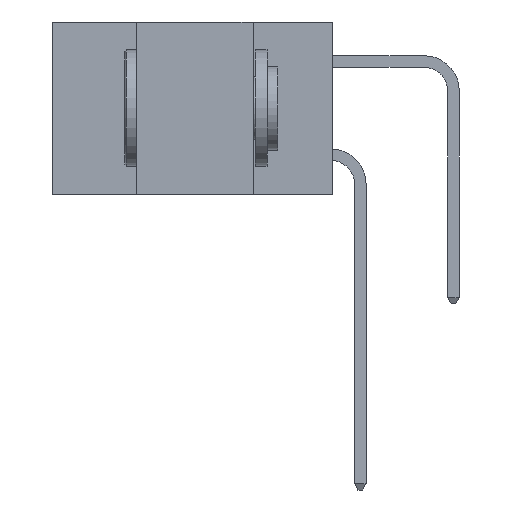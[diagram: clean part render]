
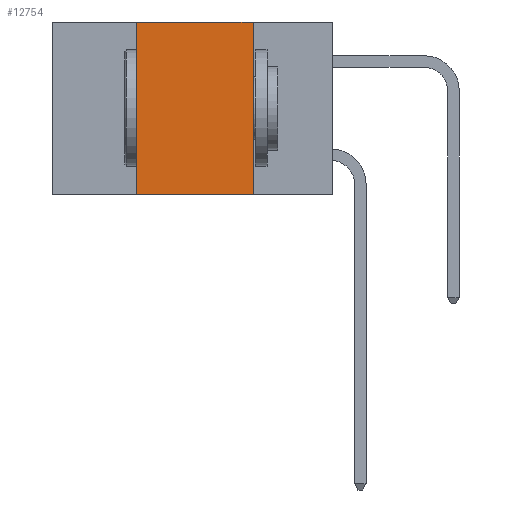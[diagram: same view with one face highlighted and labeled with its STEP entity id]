
A CAD part, left-side view. The second image highlights one B-rep face of the part: STEP entity #12754.
In plain terms, the highlighted planar face has unit normal (-1, 0, 0).
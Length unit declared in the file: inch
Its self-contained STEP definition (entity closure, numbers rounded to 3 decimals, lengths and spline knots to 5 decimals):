
#798 = EDGE_CURVE ( 'NONE', #11779, #3579, #15846, .T. ) ;
#1297 = CARTESIAN_POINT ( 'NONE',  ( 0., 0.42, -0.37 ) ) ;
#1441 = CARTESIAN_POINT ( 'NONE',  ( 0., 0.42, 0. ) ) ;
#1873 = LINE ( 'NONE', #5554, #5101 ) ;
#2264 = CARTESIAN_POINT ( 'NONE',  ( 0., 0.17, -0.37 ) ) ;
#3315 = VECTOR ( 'NONE', #6738, 39.37008 ) ;
#3579 = VERTEX_POINT ( 'NONE', #16604 ) ;
#5010 = VERTEX_POINT ( 'NONE', #7281 ) ;
#5101 = VECTOR ( 'NONE', #16122, 39.37008 ) ;
#5201 = CARTESIAN_POINT ( 'NONE',  ( 0., 0.6, 0. ) ) ;
#5554 = CARTESIAN_POINT ( 'NONE',  ( 0., 0.6, 0. ) ) ;
#5760 = LINE ( 'NONE', #1297, #12857 ) ;
#6645 = VERTEX_POINT ( 'NONE', #1441 ) ;
#6738 = DIRECTION ( 'NONE',  ( 0., -1., 0. ) ) ;
#7281 = CARTESIAN_POINT ( 'NONE',  ( 0., 0.42, -0.37 ) ) ;
#9270 = DIRECTION ( 'NONE',  ( 0., 0., -1. ) ) ;
#10250 = DIRECTION ( 'NONE',  ( 0., 0., -1. ) ) ;
#10733 = CARTESIAN_POINT ( 'NONE',  ( 0., 0.6, -0.37 ) ) ;
#10824 = DIRECTION ( 'NONE',  ( 0., 0., 1. ) ) ;
#11214 = EDGE_LOOP ( 'NONE', ( #16449, #16461, #16512, #16583 ) ) ;
#11779 = VERTEX_POINT ( 'NONE', #16746 ) ;
#12754 = ADVANCED_FACE ( 'NONE', ( #15932 ), #16987, .F. ) ;
#12857 = VECTOR ( 'NONE', #10824, 39.37008 ) ;
#12935 = EDGE_CURVE ( 'NONE', #5010, #3579, #13492, .T. ) ;
#13412 = AXIS2_PLACEMENT_3D ( 'NONE', #5201, #17036, #9270 ) ;
#13492 = LINE ( 'NONE', #10733, #3315 ) ;
#13792 = EDGE_CURVE ( 'NONE', #5010, #6645, #5760, .T. ) ;
#14668 = EDGE_CURVE ( 'NONE', #6645, #11779, #1873, .T. ) ;
#15846 = LINE ( 'NONE', #2264, #16645 ) ;
#15932 = FACE_OUTER_BOUND ( 'NONE', #11214, .T. ) ;
#16122 = DIRECTION ( 'NONE',  ( 0., -1., 0. ) ) ;
#16449 = ORIENTED_EDGE ( 'NONE', *, *, #798, .F. ) ;
#16461 = ORIENTED_EDGE ( 'NONE', *, *, #14668, .F. ) ;
#16512 = ORIENTED_EDGE ( 'NONE', *, *, #13792, .F. ) ;
#16583 = ORIENTED_EDGE ( 'NONE', *, *, #12935, .T. ) ;
#16604 = CARTESIAN_POINT ( 'NONE',  ( 0., 0.17, -0.37 ) ) ;
#16645 = VECTOR ( 'NONE', #10250, 39.37008 ) ;
#16746 = CARTESIAN_POINT ( 'NONE',  ( 0., 0.17, 0. ) ) ;
#16987 = PLANE ( 'NONE',  #13412 ) ;
#17036 = DIRECTION ( 'NONE',  ( 1., 0., 0. ) ) ;
